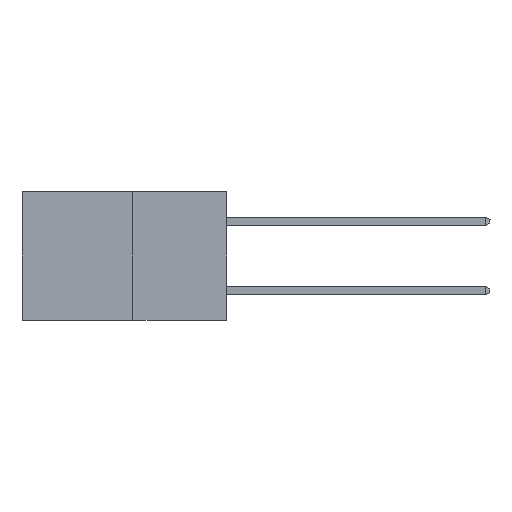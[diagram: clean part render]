
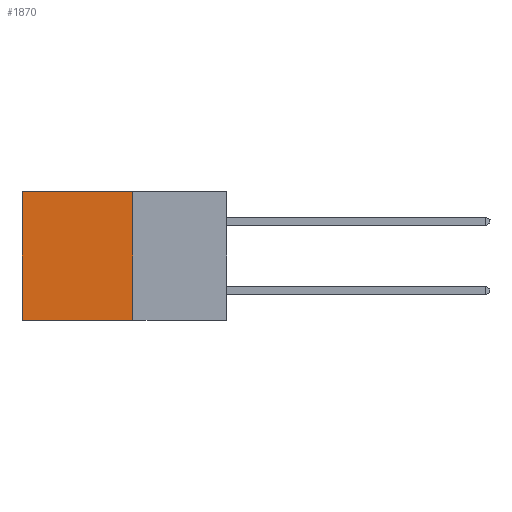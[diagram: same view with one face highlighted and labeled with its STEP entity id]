
A CAD part, left-side view. The second image highlights one B-rep face of the part: STEP entity #1870.
In plain terms, the highlighted planar face has unit normal (-1, 0, 0).
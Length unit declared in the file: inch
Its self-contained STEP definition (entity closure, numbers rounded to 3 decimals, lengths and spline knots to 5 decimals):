
#227 = EDGE_LOOP ( 'NONE', ( #1743, #4179, #3654, #1061 ) ) ;
#264 = EDGE_CURVE ( 'NONE', #2987, #2373, #10868, .T. ) ;
#708 = DIRECTION ( 'NONE',  ( 0., 1., 0. ) ) ;
#1061 = ORIENTED_EDGE ( 'NONE', *, *, #1231, .T. ) ;
#1171 = AXIS2_PLACEMENT_3D ( 'NONE', #10782, #9610, #10723 ) ;
#1231 = EDGE_CURVE ( 'NONE', #4059, #7441, #4061, .T. ) ;
#1382 = DIRECTION ( 'NONE',  ( 0., 0., -1. ) ) ;
#1743 = ORIENTED_EDGE ( 'NONE', *, *, #10716, .T. ) ;
#1870 = ADVANCED_FACE ( 'NONE', ( #7349 ), #10798, .F. ) ;
#2373 = VERTEX_POINT ( 'NONE', #4794 ) ;
#2523 = EDGE_CURVE ( 'NONE', #4059, #2987, #7572, .T. ) ;
#2775 = CARTESIAN_POINT ( 'NONE',  ( 0.277, 0.27, -0.37 ) ) ;
#2987 = VERTEX_POINT ( 'NONE', #2775 ) ;
#3153 = VECTOR ( 'NONE', #3652, 39.37008 ) ;
#3522 = VECTOR ( 'NONE', #10488, 39.37008 ) ;
#3652 = DIRECTION ( 'NONE',  ( 0., 0., -1. ) ) ;
#3654 = ORIENTED_EDGE ( 'NONE', *, *, #2523, .F. ) ;
#4059 = VERTEX_POINT ( 'NONE', #9866 ) ;
#4061 = LINE ( 'NONE', #9892, #3522 ) ;
#4179 = ORIENTED_EDGE ( 'NONE', *, *, #264, .F. ) ;
#4495 = VECTOR ( 'NONE', #708, 39.37008 ) ;
#4794 = CARTESIAN_POINT ( 'NONE',  ( 0.277, 0.59, -0.37 ) ) ;
#6458 = CARTESIAN_POINT ( 'NONE',  ( 0.277, 0.59, 0. ) ) ;
#6568 = CARTESIAN_POINT ( 'NONE',  ( 0.277, 0.27, -0.37 ) ) ;
#7349 = FACE_OUTER_BOUND ( 'NONE', #227, .T. ) ;
#7351 = LINE ( 'NONE', #8656, #3153 ) ;
#7441 = VERTEX_POINT ( 'NONE', #6458 ) ;
#7572 = LINE ( 'NONE', #10316, #8961 ) ;
#8656 = CARTESIAN_POINT ( 'NONE',  ( 0.277, 0.59, -0.37 ) ) ;
#8961 = VECTOR ( 'NONE', #1382, 39.37008 ) ;
#9610 = DIRECTION ( 'NONE',  ( 1., 0., 0. ) ) ;
#9866 = CARTESIAN_POINT ( 'NONE',  ( 0.277, 0.27, 0. ) ) ;
#9892 = CARTESIAN_POINT ( 'NONE',  ( 0.277, 0.27, 0. ) ) ;
#10316 = CARTESIAN_POINT ( 'NONE',  ( 0.277, 0.27, -0.37 ) ) ;
#10488 = DIRECTION ( 'NONE',  ( 0., 1., 0. ) ) ;
#10716 = EDGE_CURVE ( 'NONE', #7441, #2373, #7351, .T. ) ;
#10723 = DIRECTION ( 'NONE',  ( 0., 0., -1. ) ) ;
#10782 = CARTESIAN_POINT ( 'NONE',  ( 0.277, 0.27, -0.37 ) ) ;
#10798 = PLANE ( 'NONE',  #1171 ) ;
#10868 = LINE ( 'NONE', #6568, #4495 ) ;
